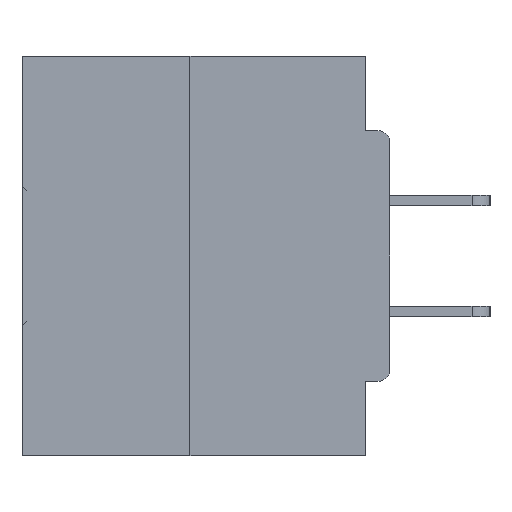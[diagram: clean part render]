
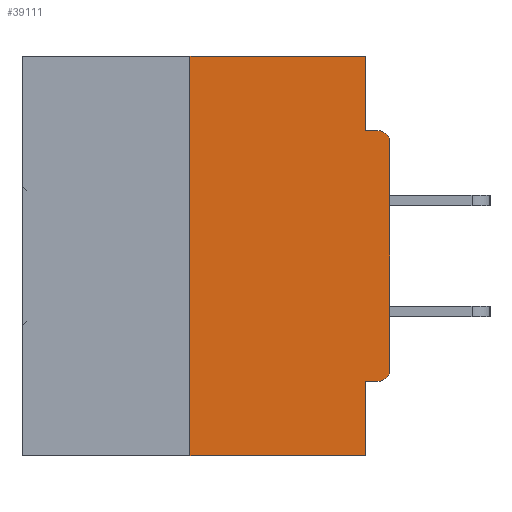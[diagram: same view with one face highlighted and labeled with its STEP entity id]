
A CAD part, left-side view. The second image highlights one B-rep face of the part: STEP entity #39111.
In plain terms, the highlighted planar face has unit normal (-1, 0, 0).
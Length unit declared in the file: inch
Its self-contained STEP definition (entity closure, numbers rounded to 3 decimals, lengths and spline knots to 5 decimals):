
#23 = VECTOR ( 'NONE', #18842, 39.37008 ) ;
#279 = EDGE_CURVE ( 'NONE', #12945, #33706, #2292, .T. ) ;
#448 = EDGE_CURVE ( 'NONE', #31946, #33706, #39122, .T. ) ;
#785 = LINE ( 'NONE', #25978, #36523 ) ;
#883 = CARTESIAN_POINT ( 'NONE',  ( 0., 0.46, -0.5 ) ) ;
#1162 = ORIENTED_EDGE ( 'NONE', *, *, #448, .F. ) ;
#1706 = VECTOR ( 'NONE', #23046, 39.37008 ) ;
#2292 = CIRCLE ( 'NONE', #36148, 0.015 ) ;
#3421 = FACE_OUTER_BOUND ( 'NONE', #3801, .T. ) ;
#3801 = EDGE_LOOP ( 'NONE', ( #12272, #39105, #18435, #9542, #7991, #22385, #16069, #20876, #1162, #9525 ) ) ;
#3980 = CARTESIAN_POINT ( 'NONE',  ( 0., 0.46, 0. ) ) ;
#4668 = VERTEX_POINT ( 'NONE', #24546 ) ;
#6164 = DIRECTION ( 'NONE',  ( -1., 0., 0. ) ) ;
#7106 = CIRCLE ( 'NONE', #38709, 0.015 ) ;
#7228 = DIRECTION ( 'NONE',  ( 0., 0., -1. ) ) ;
#7991 = ORIENTED_EDGE ( 'NONE', *, *, #16590, .F. ) ;
#8164 = VECTOR ( 'NONE', #7228, 39.37008 ) ;
#9263 = LINE ( 'NONE', #35200, #8164 ) ;
#9525 = ORIENTED_EDGE ( 'NONE', *, *, #25219, .F. ) ;
#9542 = ORIENTED_EDGE ( 'NONE', *, *, #12890, .F. ) ;
#10144 = CARTESIAN_POINT ( 'NONE',  ( 0., 0.015, -0.3915 ) ) ;
#10361 = CARTESIAN_POINT ( 'NONE',  ( 0., 0.031, -0.0935 ) ) ;
#10464 = CARTESIAN_POINT ( 'NONE',  ( 0., 0.031, -0.4065 ) ) ;
#11053 = DIRECTION ( 'NONE',  ( 0., 0., -1. ) ) ;
#11358 = PLANE ( 'NONE',  #28234 ) ;
#11533 = DIRECTION ( 'NONE',  ( 0., 0., 1. ) ) ;
#12272 = ORIENTED_EDGE ( 'NONE', *, *, #13471, .F. ) ;
#12890 = EDGE_CURVE ( 'NONE', #32845, #42136, #13862, .T. ) ;
#12945 = VERTEX_POINT ( 'NONE', #43511 ) ;
#13133 = CARTESIAN_POINT ( 'NONE',  ( 0., 0.25, 0. ) ) ;
#13471 = EDGE_CURVE ( 'NONE', #42908, #14031, #45124, .T. ) ;
#13513 = VECTOR ( 'NONE', #20164, 39.37008 ) ;
#13727 = DIRECTION ( 'NONE',  ( 0., 0., -1. ) ) ;
#13862 = LINE ( 'NONE', #39837, #23 ) ;
#14031 = VERTEX_POINT ( 'NONE', #34856 ) ;
#15416 = CARTESIAN_POINT ( 'NONE',  ( 0., 0., -0.0935 ) ) ;
#16069 = ORIENTED_EDGE ( 'NONE', *, *, #27937, .T. ) ;
#16590 = EDGE_CURVE ( 'NONE', #42914, #32845, #27317, .T. ) ;
#17425 = DIRECTION ( 'NONE',  ( 0., 0., -1. ) ) ;
#18435 = ORIENTED_EDGE ( 'NONE', *, *, #24054, .T. ) ;
#18842 = DIRECTION ( 'NONE',  ( 0., 0., -1. ) ) ;
#20164 = DIRECTION ( 'NONE',  ( 0., 0., 1. ) ) ;
#20876 = ORIENTED_EDGE ( 'NONE', *, *, #279, .T. ) ;
#21428 = CARTESIAN_POINT ( 'NONE',  ( 0., 0.25, 0. ) ) ;
#22385 = ORIENTED_EDGE ( 'NONE', *, *, #24722, .T. ) ;
#23046 = DIRECTION ( 'NONE',  ( 0., -1., 0. ) ) ;
#24054 = EDGE_CURVE ( 'NONE', #43325, #42136, #31949, .T. ) ;
#24546 = CARTESIAN_POINT ( 'NONE',  ( 0., 0., -0.3915 ) ) ;
#24722 = EDGE_CURVE ( 'NONE', #42914, #4668, #7106, .T. ) ;
#25219 = EDGE_CURVE ( 'NONE', #14031, #31946, #9263, .T. ) ;
#25978 = CARTESIAN_POINT ( 'NONE',  ( 0., 0., 0. ) ) ;
#26541 = CARTESIAN_POINT ( 'NONE',  ( 0., 0.031, -0.5 ) ) ;
#27269 = EDGE_CURVE ( 'NONE', #43325, #42908, #33824, .T. ) ;
#27317 = LINE ( 'NONE', #38585, #35525 ) ;
#27937 = EDGE_CURVE ( 'NONE', #4668, #12945, #785, .T. ) ;
#28234 = AXIS2_PLACEMENT_3D ( 'NONE', #35920, #28270, #11053 ) ;
#28270 = DIRECTION ( 'NONE',  ( 1., 0., 0. ) ) ;
#28339 = CARTESIAN_POINT ( 'NONE',  ( 0., 0.015, -0.4065 ) ) ;
#29046 = DIRECTION ( 'NONE',  ( 0., -1., 0. ) ) ;
#30906 = CARTESIAN_POINT ( 'NONE',  ( 0., 0.015, -0.1085 ) ) ;
#31946 = VERTEX_POINT ( 'NONE', #10361 ) ;
#31949 = LINE ( 'NONE', #883, #36861 ) ;
#32845 = VERTEX_POINT ( 'NONE', #10464 ) ;
#32919 = CARTESIAN_POINT ( 'NONE',  ( 0., 0.015, -0.0935 ) ) ;
#33706 = VERTEX_POINT ( 'NONE', #32919 ) ;
#33824 = LINE ( 'NONE', #13133, #13513 ) ;
#34856 = CARTESIAN_POINT ( 'NONE',  ( 0., 0.031, 0. ) ) ;
#35200 = CARTESIAN_POINT ( 'NONE',  ( 0., 0.031, 0. ) ) ;
#35525 = VECTOR ( 'NONE', #42106, 39.37008 ) ;
#35543 = CARTESIAN_POINT ( 'NONE',  ( 0., 0.25, -0.5 ) ) ;
#35767 = VECTOR ( 'NONE', #39291, 39.37008 ) ;
#35920 = CARTESIAN_POINT ( 'NONE',  ( 0., 0.46, 0. ) ) ;
#36148 = AXIS2_PLACEMENT_3D ( 'NONE', #30906, #45027, #17425 ) ;
#36523 = VECTOR ( 'NONE', #11533, 39.37008 ) ;
#36861 = VECTOR ( 'NONE', #29046, 39.37008 ) ;
#38585 = CARTESIAN_POINT ( 'NONE',  ( 0., 0., -0.4065 ) ) ;
#38709 = AXIS2_PLACEMENT_3D ( 'NONE', #10144, #6164, #13727 ) ;
#39105 = ORIENTED_EDGE ( 'NONE', *, *, #27269, .F. ) ;
#39111 = ADVANCED_FACE ( 'NONE', ( #3421 ), #11358, .F. ) ;
#39122 = LINE ( 'NONE', #15416, #1706 ) ;
#39291 = DIRECTION ( 'NONE',  ( 0., -1., 0. ) ) ;
#39837 = CARTESIAN_POINT ( 'NONE',  ( 0., 0.031, -0.5 ) ) ;
#42106 = DIRECTION ( 'NONE',  ( 0., 1., 0. ) ) ;
#42136 = VERTEX_POINT ( 'NONE', #26541 ) ;
#42908 = VERTEX_POINT ( 'NONE', #21428 ) ;
#42914 = VERTEX_POINT ( 'NONE', #28339 ) ;
#43325 = VERTEX_POINT ( 'NONE', #35543 ) ;
#43511 = CARTESIAN_POINT ( 'NONE',  ( 0., 0., -0.1085 ) ) ;
#45027 = DIRECTION ( 'NONE',  ( -1., 0., 0. ) ) ;
#45124 = LINE ( 'NONE', #3980, #35767 ) ;
